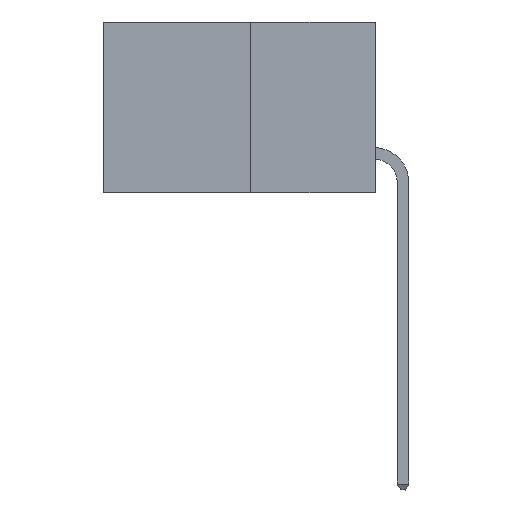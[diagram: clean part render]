
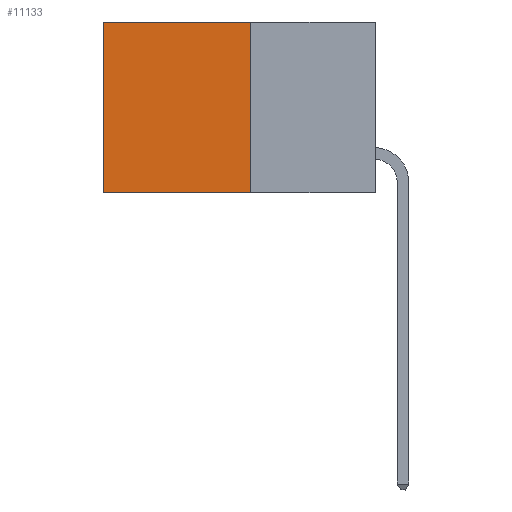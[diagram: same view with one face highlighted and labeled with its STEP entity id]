
A CAD part, left-side view. The second image highlights one B-rep face of the part: STEP entity #11133.
In plain terms, the highlighted planar face has unit normal (-1, 0, 0).
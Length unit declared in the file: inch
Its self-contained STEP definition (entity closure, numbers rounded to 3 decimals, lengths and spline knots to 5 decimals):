
#110 = VERTEX_POINT ( 'NONE', #10089 ) ;
#179 = ORIENTED_EDGE ( 'NONE', *, *, #7369, .F. ) ;
#378 = DIRECTION ( 'NONE',  ( 1., 0., 0. ) ) ;
#1227 = PLANE ( 'NONE',  #4321 ) ;
#1389 = ORIENTED_EDGE ( 'NONE', *, *, #8745, .T. ) ;
#1402 = ORIENTED_EDGE ( 'NONE', *, *, #6020, .F. ) ;
#1771 = LINE ( 'NONE', #4582, #6458 ) ;
#2344 = EDGE_LOOP ( 'NONE', ( #1389, #179, #1402, #4617 ) ) ;
#2596 = LINE ( 'NONE', #5862, #6969 ) ;
#3241 = DIRECTION ( 'NONE',  ( 0., 1., 0. ) ) ;
#3648 = CARTESIAN_POINT ( 'NONE',  ( 0.277, 0.27, 0. ) ) ;
#3747 = VECTOR ( 'NONE', #3241, 39.37008 ) ;
#3937 = FACE_OUTER_BOUND ( 'NONE', #2344, .T. ) ;
#4174 = CARTESIAN_POINT ( 'NONE',  ( 0.277, 0.27, -0.37 ) ) ;
#4321 = AXIS2_PLACEMENT_3D ( 'NONE', #5674, #378, #6543 ) ;
#4552 = DIRECTION ( 'NONE',  ( 0., 0., -1. ) ) ;
#4582 = CARTESIAN_POINT ( 'NONE',  ( 0.277, 0.59, -0.37 ) ) ;
#4617 = ORIENTED_EDGE ( 'NONE', *, *, #4710, .T. ) ;
#4710 = EDGE_CURVE ( 'NONE', #6185, #110, #6042, .T. ) ;
#5171 = VERTEX_POINT ( 'NONE', #4174 ) ;
#5602 = DIRECTION ( 'NONE',  ( 0., 0., -1. ) ) ;
#5661 = VECTOR ( 'NONE', #6929, 39.37008 ) ;
#5674 = CARTESIAN_POINT ( 'NONE',  ( 0.277, 0.27, -0.37 ) ) ;
#5862 = CARTESIAN_POINT ( 'NONE',  ( 0.277, 0.27, -0.37 ) ) ;
#6020 = EDGE_CURVE ( 'NONE', #6185, #5171, #2596, .T. ) ;
#6042 = LINE ( 'NONE', #3648, #3747 ) ;
#6185 = VERTEX_POINT ( 'NONE', #6467 ) ;
#6458 = VECTOR ( 'NONE', #4552, 39.37008 ) ;
#6467 = CARTESIAN_POINT ( 'NONE',  ( 0.277, 0.27, 0. ) ) ;
#6543 = DIRECTION ( 'NONE',  ( 0., 0., -1. ) ) ;
#6804 = CARTESIAN_POINT ( 'NONE',  ( 0.277, 0.27, -0.37 ) ) ;
#6929 = DIRECTION ( 'NONE',  ( 0., 1., 0. ) ) ;
#6969 = VECTOR ( 'NONE', #5602, 39.37008 ) ;
#7050 = CARTESIAN_POINT ( 'NONE',  ( 0.277, 0.59, -0.37 ) ) ;
#7369 = EDGE_CURVE ( 'NONE', #5171, #9151, #10160, .T. ) ;
#8745 = EDGE_CURVE ( 'NONE', #110, #9151, #1771, .T. ) ;
#9151 = VERTEX_POINT ( 'NONE', #7050 ) ;
#10089 = CARTESIAN_POINT ( 'NONE',  ( 0.277, 0.59, 0. ) ) ;
#10160 = LINE ( 'NONE', #6804, #5661 ) ;
#11133 = ADVANCED_FACE ( 'NONE', ( #3937 ), #1227, .F. ) ;
